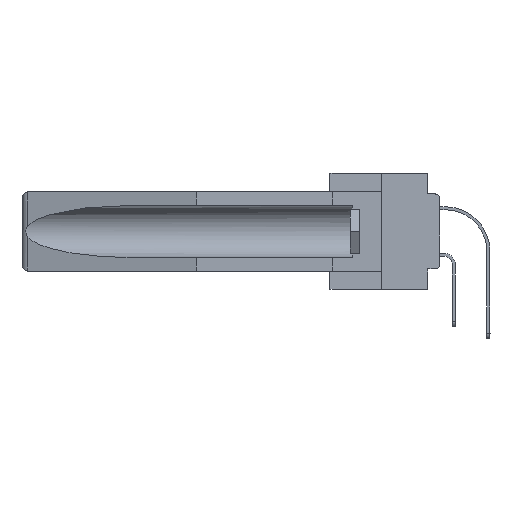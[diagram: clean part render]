
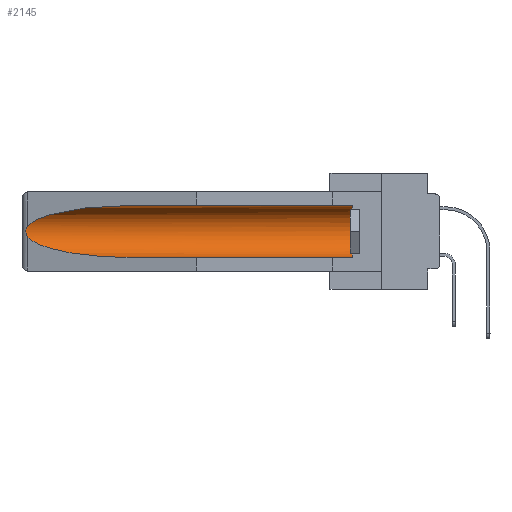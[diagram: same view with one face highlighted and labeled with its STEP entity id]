
A CAD part, left-side view. The second image highlights one B-rep face of the part: STEP entity #2145.
In plain terms, the highlighted cylindrical face has radius 2.857 mm (diameter 5.715 mm), a partial arc.
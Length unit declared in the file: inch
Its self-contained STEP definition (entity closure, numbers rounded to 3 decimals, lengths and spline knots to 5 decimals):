
#75 = CARTESIAN_POINT ( 'NONE',  ( 0.155, 1.07973, -0.059 ) ) ;
#315 = CARTESIAN_POINT ( 'NONE',  ( 0.2673, 1.5327, -0.16383 ) ) ;
#591 = CARTESIAN_POINT ( 'NONE',  ( 0.155, 1.07973, -0.059 ) ) ;
#2145 = ADVANCED_FACE ( 'NONE', ( #25212 ), #2774, .F. ) ;
#2774 = CYLINDRICAL_SURFACE ( 'NONE', #32773, 0.1125 ) ;
#3045 = CIRCLE ( 'NONE', #4222, 0.1125 ) ;
#3270 = CARTESIAN_POINT ( 'NONE',  ( 0.26597, 1.5296, -0.19026 ) ) ;
#4222 = AXIS2_PLACEMENT_3D ( 'NONE', #24654, #36018, #26908 ) ;
#4317 = EDGE_CURVE ( 'NONE', #5328, #35593, #3045, .T. ) ;
#4512 = CARTESIAN_POINT ( 'NONE',  ( 0.26537, 1.52718, -0.14972 ) ) ;
#4996 = CARTESIAN_POINT ( 'NONE',  ( 0.155, -0.30754, -0.1715 ) ) ;
#5328 = VERTEX_POINT ( 'NONE', #24563 ) ;
#5457 = EDGE_CURVE ( 'NONE', #35593, #22352, #25488, .T. ) ;
#5875 = CARTESIAN_POINT ( 'NONE',  ( 0.26537, 1.52718, -0.19328 ) ) ;
#6124 = CARTESIAN_POINT ( 'NONE',  ( 0.25451, 1.48313, -0.09465 ) ) ;
#7435 = LINE ( 'NONE', #23774, #23399 ) ;
#8872 = ORIENTED_EDGE ( 'NONE', *, *, #26591, .T. ) ;
#8908 = B_SPLINE_CURVE_WITH_KNOTS ( 'NONE', 3,
 ( #20495, #14005, #19728, #315, #11231, #25352, #28705, #25901, #3270, #5875 ),
 .UNSPECIFIED., .F., .F.,
 ( 4, 2, 2, 2, 4 ),
 ( 0., 0.00029, 0.00058, 0.00087, 0.00117 ),
 .UNSPECIFIED. ) ;
#9218 = EDGE_LOOP ( 'NONE', ( #23309, #8872, #23727, #9394, #9957, #36167 ) ) ;
#9394 = ORIENTED_EDGE ( 'NONE', *, *, #19474, .F. ) ;
#9791 = CARTESIAN_POINT ( 'NONE',  ( 0.155, 1.07973, -0.284 ) ) ;
#9957 = ORIENTED_EDGE ( 'NONE', *, *, #4317, .T. ) ;
#11231 = CARTESIAN_POINT ( 'NONE',  ( 0.2675, 1.53308, -0.16763 ) ) ;
#12810 = DIRECTION ( 'NONE',  ( 0., 1., 0. ) ) ;
#14005 = CARTESIAN_POINT ( 'NONE',  ( 0.26597, 1.52961, -0.15275 ) ) ;
#14331 =( BOUNDED_CURVE ( )  B_SPLINE_CURVE ( 3, ( #35255, #32835, #30038, #9791 ),
 .UNSPECIFIED., .F., .T. ) 
 B_SPLINE_CURVE_WITH_KNOTS ( ( 4, 4 ),
 ( 0.1948, 1.5708 ),
 .UNSPECIFIED. ) 
 CURVE ( )  GEOMETRIC_REPRESENTATION_ITEM ( )  RATIONAL_B_SPLINE_CURVE ( ( 1., 0.848, 0.848, 1. ) ) 
 REPRESENTATION_ITEM ( '' )  );
#17868 = CARTESIAN_POINT ( 'NONE',  ( 0.26537, 1.52718, -0.19328 ) ) ;
#19474 = EDGE_CURVE ( 'NONE', #5328, #35354, #7435, .T. ) ;
#19728 = CARTESIAN_POINT ( 'NONE',  ( 0.26654, 1.53092, -0.15636 ) ) ;
#20495 = CARTESIAN_POINT ( 'NONE',  ( 0.26537, 1.52718, -0.14972 ) ) ;
#20912 = CARTESIAN_POINT ( 'NONE',  ( 0.155, 0.126, -0.059 ) ) ;
#22242 = DIRECTION ( 'NONE',  ( 0., 1., 0. ) ) ;
#22352 = VERTEX_POINT ( 'NONE', #75 ) ;
#23309 = ORIENTED_EDGE ( 'NONE', *, *, #30942, .T. ) ;
#23399 = VECTOR ( 'NONE', #12810, 39.37008 ) ;
#23727 = ORIENTED_EDGE ( 'NONE', *, *, #27509, .T. ) ;
#23774 = CARTESIAN_POINT ( 'NONE',  ( 0.155, -0.30754, -0.284 ) ) ;
#24563 = CARTESIAN_POINT ( 'NONE',  ( 0.155, 0.126, -0.284 ) ) ;
#24654 = CARTESIAN_POINT ( 'NONE',  ( 0.155, 0.126, -0.1715 ) ) ;
#25212 = FACE_OUTER_BOUND ( 'NONE', #9218, .T. ) ;
#25352 = CARTESIAN_POINT ( 'NONE',  ( 0.2675, 1.53308, -0.17534 ) ) ;
#25415 = VERTEX_POINT ( 'NONE', #17868 ) ;
#25488 = LINE ( 'NONE', #34057, #36301 ) ;
#25901 = CARTESIAN_POINT ( 'NONE',  ( 0.26655, 1.53094, -0.18657 ) ) ;
#26316 = CARTESIAN_POINT ( 'NONE',  ( 0.155, 1.07973, -0.284 ) ) ;
#26591 = EDGE_CURVE ( 'NONE', #27292, #25415, #8908, .T. ) ;
#26908 = DIRECTION ( 'NONE',  ( 0., 0., 1. ) ) ;
#27292 = VERTEX_POINT ( 'NONE', #4512 ) ;
#27509 = EDGE_CURVE ( 'NONE', #25415, #35354, #14331, .T. ) ;
#28705 = CARTESIAN_POINT ( 'NONE',  ( 0.2673, 1.53269, -0.17917 ) ) ;
#29550 =( BOUNDED_CURVE ( )  B_SPLINE_CURVE ( 3, ( #591, #34545, #6124, #32128 ),
 .UNSPECIFIED., .F., .T. ) 
 B_SPLINE_CURVE_WITH_KNOTS ( ( 4, 4 ),
 ( 4.71239, 6.08839 ),
 .UNSPECIFIED. ) 
 CURVE ( )  GEOMETRIC_REPRESENTATION_ITEM ( )  RATIONAL_B_SPLINE_CURVE ( ( 1., 0.848, 0.848, 1. ) ) 
 REPRESENTATION_ITEM ( '' )  );
#30038 = CARTESIAN_POINT ( 'NONE',  ( 0.21114, 1.30732, -0.284 ) ) ;
#30942 = EDGE_CURVE ( 'NONE', #22352, #27292, #29550, .T. ) ;
#31454 = DIRECTION ( 'NONE',  ( 0., 1., 0. ) ) ;
#32128 = CARTESIAN_POINT ( 'NONE',  ( 0.26537, 1.52718, -0.14972 ) ) ;
#32773 = AXIS2_PLACEMENT_3D ( 'NONE', #4996, #22242, #36199 ) ;
#32835 = CARTESIAN_POINT ( 'NONE',  ( 0.25451, 1.48313, -0.24835 ) ) ;
#34057 = CARTESIAN_POINT ( 'NONE',  ( 0.155, -0.30754, -0.059 ) ) ;
#34545 = CARTESIAN_POINT ( 'NONE',  ( 0.21114, 1.30732, -0.059 ) ) ;
#35255 = CARTESIAN_POINT ( 'NONE',  ( 0.26537, 1.52718, -0.19328 ) ) ;
#35354 = VERTEX_POINT ( 'NONE', #26316 ) ;
#35593 = VERTEX_POINT ( 'NONE', #20912 ) ;
#36018 = DIRECTION ( 'NONE',  ( 0., -1., 0. ) ) ;
#36167 = ORIENTED_EDGE ( 'NONE', *, *, #5457, .T. ) ;
#36199 = DIRECTION ( 'NONE',  ( 0., 0., 1. ) ) ;
#36301 = VECTOR ( 'NONE', #31454, 39.37008 ) ;
